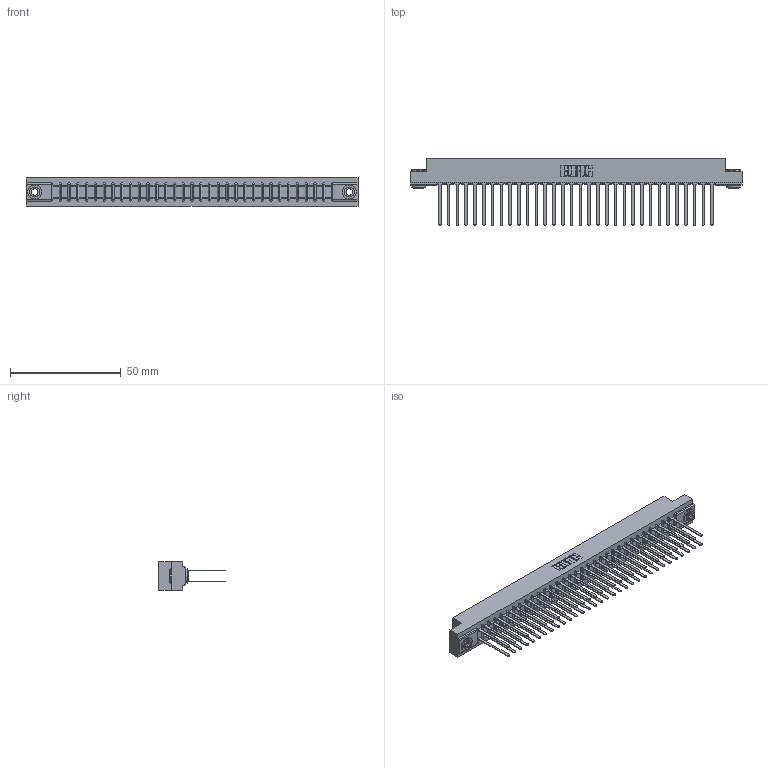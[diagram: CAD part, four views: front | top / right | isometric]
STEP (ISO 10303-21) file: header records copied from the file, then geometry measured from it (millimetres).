
FILE_DESCRIPTION (( 'STEP AP203' ), '1' );
FILE_NAME ('357-064-540-203.STEP', '2018-08-12T16:24:04', ( '' ), ( '' ), 'SwSTEP 2.0', 'SolidWorks 2016', '' );
FILE_SCHEMA (( 'CONFIG_CONTROL_DESIGN' ));
Length unit declared in the file: inch
Products named in the file (4): 307 Part_.156 Dia Mounting Holes; 307-290-001_540; 345-250-002_345-250-002-102; 357-064-540-203
Assembly tree (67 placements, depth 2):
  357-064-540-203
    307 Part_.156 Dia Mounting Holes
    307-290-001_540  x64
    345-250-002_345-250-002-102  x2
Bounding box: 149.81 x 30 x 12.7 mm (x, y, z)
Volume: 16218.2 mm3; surface area: 22027.3 mm2
Topology: 67 solids, 67 shells, 3147 faces, 8755 edges, 5658 vertices
Faces by surface type: plane 2078, cylinder 995, sphere 66, cone 8
Entity records: 30723 total; most frequent: CARTESIAN_POINT 5009, ORIENTED_EDGE 4954, DIRECTION 4925, EDGE_CURVE 2477, VECTOR 1889, LINE 1889, VERTEX_POINT 1602, AXIS2_PLACEMENT_3D 1518
